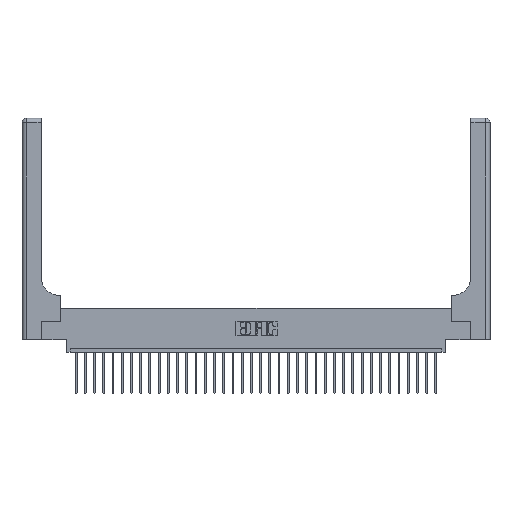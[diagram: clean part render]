
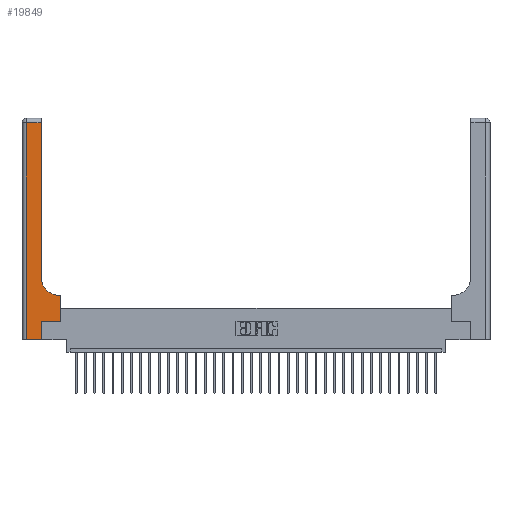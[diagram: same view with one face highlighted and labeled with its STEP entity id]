
A CAD part, top view. The second image highlights one B-rep face of the part: STEP entity #19849.
In plain terms, the highlighted planar face has unit normal (0, 0, 1).
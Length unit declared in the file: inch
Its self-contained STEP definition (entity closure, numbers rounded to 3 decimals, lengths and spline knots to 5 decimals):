
#53 = CARTESIAN_POINT ( 'NONE',  ( 0.265, 0.25, 0.37 ) ) ;
#80 = CARTESIAN_POINT ( 'NONE',  ( 0.528, 0.6, 0.37 ) ) ;
#103 = VECTOR ( 'NONE', #25686, 39.37008 ) ;
#757 = CARTESIAN_POINT ( 'NONE',  ( 0.06, 2.94, 0.37 ) ) ;
#894 = DIRECTION ( 'NONE',  ( 1., 0., 0. ) ) ;
#1280 = LINE ( 'NONE', #27696, #8026 ) ;
#2311 = DIRECTION ( 'NONE',  ( -1., 0., 0. ) ) ;
#2860 = CARTESIAN_POINT ( 'NONE',  ( 0.26, 2.94, 0.37 ) ) ;
#3351 = EDGE_CURVE ( 'NONE', #7561, #9775, #11293, .T. ) ;
#4695 = AXIS2_PLACEMENT_3D ( 'NONE', #21026, #13778, #30489 ) ;
#4831 = DIRECTION ( 'NONE',  ( 0., 0., -1. ) ) ;
#5318 = EDGE_CURVE ( 'NONE', #16474, #28851, #8030, .T. ) ;
#6543 = ORIENTED_EDGE ( 'NONE', *, *, #13310, .T. ) ;
#6819 = EDGE_CURVE ( 'NONE', #19246, #18610, #9687, .T. ) ;
#7281 = ORIENTED_EDGE ( 'NONE', *, *, #30726, .T. ) ;
#7561 = VERTEX_POINT ( 'NONE', #757 ) ;
#8026 = VECTOR ( 'NONE', #13481, 39.37008 ) ;
#8030 = LINE ( 'NONE', #24613, #29695 ) ;
#8312 = ORIENTED_EDGE ( 'NONE', *, *, #5318, .T. ) ;
#9065 = FACE_OUTER_BOUND ( 'NONE', #15259, .T. ) ;
#9687 = LINE ( 'NONE', #19243, #25490 ) ;
#9775 = VERTEX_POINT ( 'NONE', #19533 ) ;
#9993 = LINE ( 'NONE', #29181, #29835 ) ;
#10604 = DIRECTION ( 'NONE',  ( 0., 1., 0. ) ) ;
#11293 = LINE ( 'NONE', #30343, #103 ) ;
#11925 = AXIS2_PLACEMENT_3D ( 'NONE', #23619, #4831, #2311 ) ;
#12868 = ORIENTED_EDGE ( 'NONE', *, *, #26529, .T. ) ;
#13310 = EDGE_CURVE ( 'NONE', #30502, #25029, #9993, .T. ) ;
#13481 = DIRECTION ( 'NONE',  ( 1., 0., 0. ) ) ;
#13778 = DIRECTION ( 'NONE',  ( 0., 0., -1. ) ) ;
#13848 = ORIENTED_EDGE ( 'NONE', *, *, #27205, .T. ) ;
#14477 = VECTOR ( 'NONE', #10604, 39.37008 ) ;
#15229 = DIRECTION ( 'NONE',  ( 0., 1., 0. ) ) ;
#15259 = EDGE_LOOP ( 'NONE', ( #8312, #12868, #27515, #13848, #23637, #6543, #23429, #23452, #7281 ) ) ;
#16383 = LINE ( 'NONE', #24183, #28866 ) ;
#16474 = VERTEX_POINT ( 'NONE', #27394 ) ;
#17961 = CARTESIAN_POINT ( 'NONE',  ( 0.528, 0.25, 0.37 ) ) ;
#18447 = CARTESIAN_POINT ( 'NONE',  ( 0.51, 0.6, 0.37 ) ) ;
#18448 = VECTOR ( 'NONE', #23162, 39.37008 ) ;
#18610 = VERTEX_POINT ( 'NONE', #18447 ) ;
#19108 = CARTESIAN_POINT ( 'NONE',  ( 0.265, 0., 0.37 ) ) ;
#19243 = CARTESIAN_POINT ( 'NONE',  ( 0.26, 0.6, 0.37 ) ) ;
#19246 = VERTEX_POINT ( 'NONE', #80 ) ;
#19533 = CARTESIAN_POINT ( 'NONE',  ( 0.06, 0., 0.37 ) ) ;
#19738 = EDGE_CURVE ( 'NONE', #24333, #30502, #29983, .T. ) ;
#19849 = ADVANCED_FACE ( 'NONE', ( #9065 ), #21601, .F. ) ;
#20666 = LINE ( 'NONE', #29501, #14477 ) ;
#20840 = EDGE_CURVE ( 'NONE', #25029, #19246, #20666, .T. ) ;
#21026 = CARTESIAN_POINT ( 'NONE',  ( 0.51, 0.85, 0.37 ) ) ;
#21601 = PLANE ( 'NONE',  #11925 ) ;
#23162 = DIRECTION ( 'NONE',  ( 0., 1., 0. ) ) ;
#23429 = ORIENTED_EDGE ( 'NONE', *, *, #20840, .T. ) ;
#23452 = ORIENTED_EDGE ( 'NONE', *, *, #6819, .T. ) ;
#23619 = CARTESIAN_POINT ( 'NONE',  ( 0., 3., 0.37 ) ) ;
#23637 = ORIENTED_EDGE ( 'NONE', *, *, #19738, .T. ) ;
#24183 = CARTESIAN_POINT ( 'NONE',  ( 0., 2.94, 0.37 ) ) ;
#24333 = VERTEX_POINT ( 'NONE', #19108 ) ;
#24613 = CARTESIAN_POINT ( 'NONE',  ( 0.26, 3., 0.37 ) ) ;
#25029 = VERTEX_POINT ( 'NONE', #17961 ) ;
#25490 = VECTOR ( 'NONE', #28726, 39.37008 ) ;
#25686 = DIRECTION ( 'NONE',  ( 0., -1., 0. ) ) ;
#25924 = DIRECTION ( 'NONE',  ( -1., 0., 0. ) ) ;
#26230 = CIRCLE ( 'NONE', #4695, 0.25 ) ;
#26529 = EDGE_CURVE ( 'NONE', #28851, #7561, #16383, .T. ) ;
#27205 = EDGE_CURVE ( 'NONE', #9775, #24333, #1280, .T. ) ;
#27337 = CARTESIAN_POINT ( 'NONE',  ( 0.265, 0., 0.37 ) ) ;
#27394 = CARTESIAN_POINT ( 'NONE',  ( 0.26, 0.85, 0.37 ) ) ;
#27515 = ORIENTED_EDGE ( 'NONE', *, *, #3351, .T. ) ;
#27696 = CARTESIAN_POINT ( 'NONE',  ( 0., 0., 0.37 ) ) ;
#28726 = DIRECTION ( 'NONE',  ( -1., 0., 0. ) ) ;
#28851 = VERTEX_POINT ( 'NONE', #2860 ) ;
#28866 = VECTOR ( 'NONE', #25924, 39.37008 ) ;
#29181 = CARTESIAN_POINT ( 'NONE',  ( 0.265, 0.25, 0.37 ) ) ;
#29501 = CARTESIAN_POINT ( 'NONE',  ( 0.528, 0.25, 0.37 ) ) ;
#29695 = VECTOR ( 'NONE', #15229, 39.37008 ) ;
#29835 = VECTOR ( 'NONE', #894, 39.37008 ) ;
#29983 = LINE ( 'NONE', #27337, #18448 ) ;
#30343 = CARTESIAN_POINT ( 'NONE',  ( 0.06, 3., 0.37 ) ) ;
#30489 = DIRECTION ( 'NONE',  ( 1., 0., 0. ) ) ;
#30502 = VERTEX_POINT ( 'NONE', #53 ) ;
#30726 = EDGE_CURVE ( 'NONE', #18610, #16474, #26230, .T. ) ;
